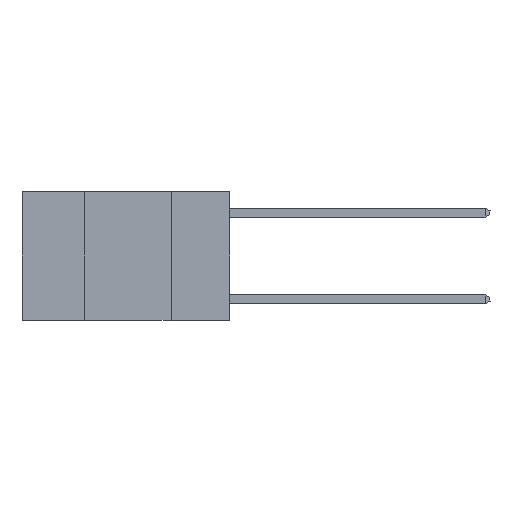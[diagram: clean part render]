
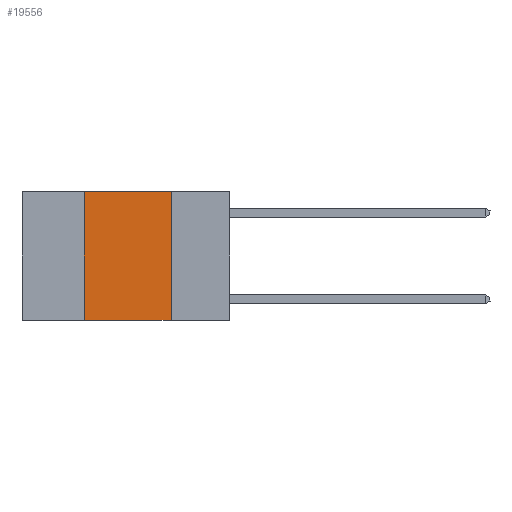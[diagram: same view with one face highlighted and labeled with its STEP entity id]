
A CAD part, left-side view. The second image highlights one B-rep face of the part: STEP entity #19556.
In plain terms, the highlighted planar face has unit normal (-1, 0, 0).
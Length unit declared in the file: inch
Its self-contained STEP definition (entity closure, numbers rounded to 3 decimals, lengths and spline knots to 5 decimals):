
#45 = FACE_OUTER_BOUND ( 'NONE', #27694, .T. ) ;
#177 = CARTESIAN_POINT ( 'NONE',  ( 0., 0.42, -0.37 ) ) ;
#639 = ORIENTED_EDGE ( 'NONE', *, *, #13175, .F. ) ;
#1516 = DIRECTION ( 'NONE',  ( 0., 0., -1. ) ) ;
#2949 = CARTESIAN_POINT ( 'NONE',  ( 0., 0.6, -0.37 ) ) ;
#3363 = LINE ( 'NONE', #17529, #25846 ) ;
#4618 = CARTESIAN_POINT ( 'NONE',  ( 0., 0.17, 0. ) ) ;
#4791 = LINE ( 'NONE', #2949, #28724 ) ;
#6030 = EDGE_CURVE ( 'NONE', #15725, #24080, #10434, .T. ) ;
#7365 = ORIENTED_EDGE ( 'NONE', *, *, #6030, .F. ) ;
#7671 = DIRECTION ( 'NONE',  ( 0., -1., 0. ) ) ;
#8150 = CARTESIAN_POINT ( 'NONE',  ( 0., 0.6, 0. ) ) ;
#8931 = VERTEX_POINT ( 'NONE', #177 ) ;
#9824 = ORIENTED_EDGE ( 'NONE', *, *, #25477, .T. ) ;
#10434 = LINE ( 'NONE', #8150, #21671 ) ;
#10678 = DIRECTION ( 'NONE',  ( 0., 0., 1. ) ) ;
#12431 = DIRECTION ( 'NONE',  ( 0., 0., -1. ) ) ;
#13175 = EDGE_CURVE ( 'NONE', #24080, #14303, #17158, .T. ) ;
#13391 = DIRECTION ( 'NONE',  ( 1., 0., 0. ) ) ;
#14303 = VERTEX_POINT ( 'NONE', #29368 ) ;
#15725 = VERTEX_POINT ( 'NONE', #26210 ) ;
#17158 = LINE ( 'NONE', #26448, #26755 ) ;
#17529 = CARTESIAN_POINT ( 'NONE',  ( 0., 0.42, 0. ) ) ;
#18635 = PLANE ( 'NONE',  #24179 ) ;
#19556 = ADVANCED_FACE ( 'NONE', ( #45 ), #18635, .F. ) ;
#21098 = ORIENTED_EDGE ( 'NONE', *, *, #26047, .F. ) ;
#21671 = VECTOR ( 'NONE', #24159, 39.37008 ) ;
#24080 = VERTEX_POINT ( 'NONE', #4618 ) ;
#24159 = DIRECTION ( 'NONE',  ( 0., -1., 0. ) ) ;
#24179 = AXIS2_PLACEMENT_3D ( 'NONE', #27942, #13391, #1516 ) ;
#25477 = EDGE_CURVE ( 'NONE', #8931, #14303, #4791, .T. ) ;
#25846 = VECTOR ( 'NONE', #10678, 39.37008 ) ;
#26047 = EDGE_CURVE ( 'NONE', #8931, #15725, #3363, .T. ) ;
#26210 = CARTESIAN_POINT ( 'NONE',  ( 0., 0.42, 0. ) ) ;
#26448 = CARTESIAN_POINT ( 'NONE',  ( 0., 0.17, 0. ) ) ;
#26755 = VECTOR ( 'NONE', #12431, 39.37008 ) ;
#27694 = EDGE_LOOP ( 'NONE', ( #639, #7365, #21098, #9824 ) ) ;
#27942 = CARTESIAN_POINT ( 'NONE',  ( 0., 0.6, 0. ) ) ;
#28724 = VECTOR ( 'NONE', #7671, 39.37008 ) ;
#29368 = CARTESIAN_POINT ( 'NONE',  ( 0., 0.17, -0.37 ) ) ;
